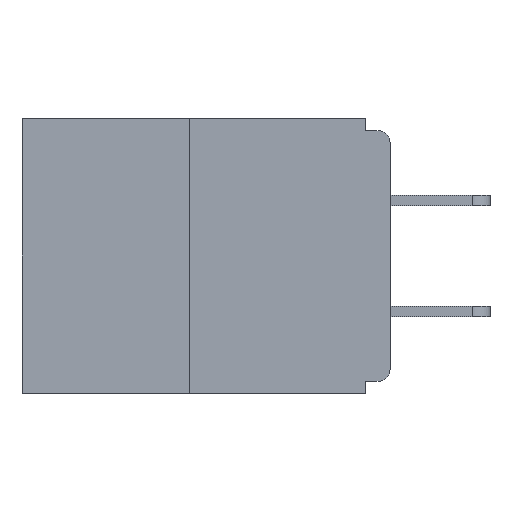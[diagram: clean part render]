
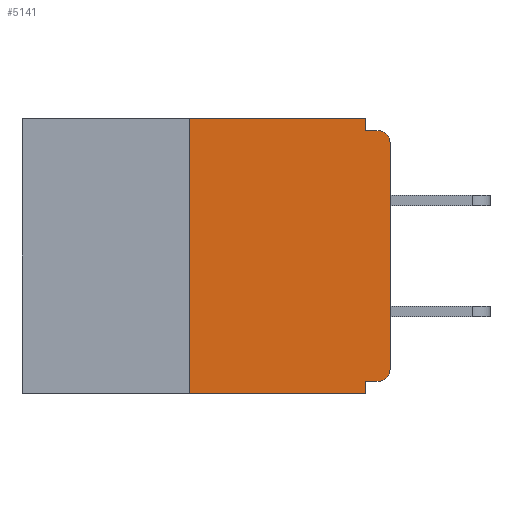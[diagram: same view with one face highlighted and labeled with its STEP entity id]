
A CAD part, left-side view. The second image highlights one B-rep face of the part: STEP entity #5141.
In plain terms, the highlighted planar face has unit normal (-1, 0, 0).
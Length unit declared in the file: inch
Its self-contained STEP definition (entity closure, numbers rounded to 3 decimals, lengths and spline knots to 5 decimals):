
#164 = CARTESIAN_POINT ( 'NONE',  ( 0., 0., -0.03 ) ) ;
#286 = EDGE_CURVE ( 'NONE', #2917, #7035, #8710, .T. ) ;
#323 = VECTOR ( 'NONE', #6793, 39.37008 ) ;
#348 = DIRECTION ( 'NONE',  ( 0., 0., 1. ) ) ;
#508 = CARTESIAN_POINT ( 'NONE',  ( 0., 0.031, 0. ) ) ;
#575 = ORIENTED_EDGE ( 'NONE', *, *, #11843, .F. ) ;
#628 = CARTESIAN_POINT ( 'NONE',  ( 0., 0.015, -0.328 ) ) ;
#1298 = CARTESIAN_POINT ( 'NONE',  ( 0., 0., 0. ) ) ;
#1333 = PLANE ( 'NONE',  #3603 ) ;
#1447 = ORIENTED_EDGE ( 'NONE', *, *, #7355, .T. ) ;
#1562 = CARTESIAN_POINT ( 'NONE',  ( 0., 0.015, -0.03 ) ) ;
#1610 = LINE ( 'NONE', #11660, #11143 ) ;
#1811 = CARTESIAN_POINT ( 'NONE',  ( 0., 0.031, -0.343 ) ) ;
#2059 = EDGE_CURVE ( 'NONE', #9774, #7039, #3763, .T. ) ;
#2115 = CARTESIAN_POINT ( 'NONE',  ( 0., 0.031, 0. ) ) ;
#2211 = VECTOR ( 'NONE', #3995, 39.37008 ) ;
#2231 = LINE ( 'NONE', #5839, #9585 ) ;
#2387 = VECTOR ( 'NONE', #348, 39.37008 ) ;
#2437 = ORIENTED_EDGE ( 'NONE', *, *, #11403, .T. ) ;
#2637 = CARTESIAN_POINT ( 'NONE',  ( 0., 0.25, -0.343 ) ) ;
#2664 = EDGE_CURVE ( 'NONE', #8603, #4849, #9278, .T. ) ;
#2917 = VERTEX_POINT ( 'NONE', #8668 ) ;
#2920 = CIRCLE ( 'NONE', #11865, 0.015 ) ;
#2966 = EDGE_CURVE ( 'NONE', #8305, #11521, #2920, .T. ) ;
#3420 = DIRECTION ( 'NONE',  ( 0., 0., 1. ) ) ;
#3603 = AXIS2_PLACEMENT_3D ( 'NONE', #4235, #10566, #8714 ) ;
#3763 = LINE ( 'NONE', #1811, #8663 ) ;
#3995 = DIRECTION ( 'NONE',  ( 0., -1., 0. ) ) ;
#4070 = DIRECTION ( 'NONE',  ( 0., 1., 0. ) ) ;
#4235 = CARTESIAN_POINT ( 'NONE',  ( 0., 0.46, 0. ) ) ;
#4272 = DIRECTION ( 'NONE',  ( -1., 0., 0. ) ) ;
#4301 = CARTESIAN_POINT ( 'NONE',  ( 0., 0.015, -0.015 ) ) ;
#4647 = DIRECTION ( 'NONE',  ( 0., 0., -1. ) ) ;
#4849 = VERTEX_POINT ( 'NONE', #7370 ) ;
#5044 = VERTEX_POINT ( 'NONE', #11350 ) ;
#5141 = ADVANCED_FACE ( 'NONE', ( #6765 ), #1333, .F. ) ;
#5597 = DIRECTION ( 'NONE',  ( 0., -1., 0. ) ) ;
#5686 = VECTOR ( 'NONE', #5597, 39.37008 ) ;
#5736 = DIRECTION ( 'NONE',  ( -1., 0., 0. ) ) ;
#5839 = CARTESIAN_POINT ( 'NONE',  ( 0., 0., -0.328 ) ) ;
#5921 = ORIENTED_EDGE ( 'NONE', *, *, #2664, .T. ) ;
#5946 = ORIENTED_EDGE ( 'NONE', *, *, #2966, .T. ) ;
#6173 = ORIENTED_EDGE ( 'NONE', *, *, #9815, .F. ) ;
#6765 = FACE_OUTER_BOUND ( 'NONE', #7159, .T. ) ;
#6793 = DIRECTION ( 'NONE',  ( 0., 0., -1. ) ) ;
#7035 = VERTEX_POINT ( 'NONE', #508 ) ;
#7039 = VERTEX_POINT ( 'NONE', #10423 ) ;
#7143 = CARTESIAN_POINT ( 'NONE',  ( 0., 0.25, 0. ) ) ;
#7159 = EDGE_LOOP ( 'NONE', ( #10808, #6173, #2437, #8590, #9526, #5921, #1447, #5946, #11519, #575 ) ) ;
#7240 = LINE ( 'NONE', #2115, #323 ) ;
#7255 = LINE ( 'NONE', #9404, #2211 ) ;
#7355 = EDGE_CURVE ( 'NONE', #4849, #8305, #8299, .T. ) ;
#7370 = CARTESIAN_POINT ( 'NONE',  ( 0., 0., -0.313 ) ) ;
#7716 = VECTOR ( 'NONE', #3420, 39.37008 ) ;
#8299 = LINE ( 'NONE', #1298, #2387 ) ;
#8305 = VERTEX_POINT ( 'NONE', #164 ) ;
#8590 = ORIENTED_EDGE ( 'NONE', *, *, #2059, .F. ) ;
#8603 = VERTEX_POINT ( 'NONE', #628 ) ;
#8625 = DIRECTION ( 'NONE',  ( 0., 0., -1. ) ) ;
#8663 = VECTOR ( 'NONE', #4647, 39.37008 ) ;
#8668 = CARTESIAN_POINT ( 'NONE',  ( 0., 0.25, 0. ) ) ;
#8710 = LINE ( 'NONE', #9144, #5686 ) ;
#8714 = DIRECTION ( 'NONE',  ( 0., 0., -1. ) ) ;
#8861 = CARTESIAN_POINT ( 'NONE',  ( 0., 0.031, -0.328 ) ) ;
#9144 = CARTESIAN_POINT ( 'NONE',  ( 0., 0.46, 0. ) ) ;
#9278 = CIRCLE ( 'NONE', #9621, 0.015 ) ;
#9370 = VERTEX_POINT ( 'NONE', #2637 ) ;
#9404 = CARTESIAN_POINT ( 'NONE',  ( 0., 0., -0.015 ) ) ;
#9526 = ORIENTED_EDGE ( 'NONE', *, *, #10172, .F. ) ;
#9585 = VECTOR ( 'NONE', #4070, 39.37008 ) ;
#9621 = AXIS2_PLACEMENT_3D ( 'NONE', #10368, #5736, #8625 ) ;
#9774 = VERTEX_POINT ( 'NONE', #8861 ) ;
#9815 = EDGE_CURVE ( 'NONE', #9370, #2917, #10020, .T. ) ;
#9860 = DIRECTION ( 'NONE',  ( 0., -1., 0. ) ) ;
#10020 = LINE ( 'NONE', #7143, #7716 ) ;
#10172 = EDGE_CURVE ( 'NONE', #8603, #9774, #2231, .T. ) ;
#10368 = CARTESIAN_POINT ( 'NONE',  ( 0., 0.015, -0.313 ) ) ;
#10423 = CARTESIAN_POINT ( 'NONE',  ( 0., 0.031, -0.343 ) ) ;
#10566 = DIRECTION ( 'NONE',  ( 1., 0., 0. ) ) ;
#10799 = DIRECTION ( 'NONE',  ( 0., 0., -1. ) ) ;
#10808 = ORIENTED_EDGE ( 'NONE', *, *, #286, .F. ) ;
#11143 = VECTOR ( 'NONE', #9860, 39.37008 ) ;
#11150 = EDGE_CURVE ( 'NONE', #5044, #11521, #7255, .T. ) ;
#11350 = CARTESIAN_POINT ( 'NONE',  ( 0., 0.031, -0.015 ) ) ;
#11403 = EDGE_CURVE ( 'NONE', #9370, #7039, #1610, .T. ) ;
#11519 = ORIENTED_EDGE ( 'NONE', *, *, #11150, .F. ) ;
#11521 = VERTEX_POINT ( 'NONE', #4301 ) ;
#11660 = CARTESIAN_POINT ( 'NONE',  ( 0., 0.46, -0.343 ) ) ;
#11843 = EDGE_CURVE ( 'NONE', #7035, #5044, #7240, .T. ) ;
#11865 = AXIS2_PLACEMENT_3D ( 'NONE', #1562, #4272, #10799 ) ;
